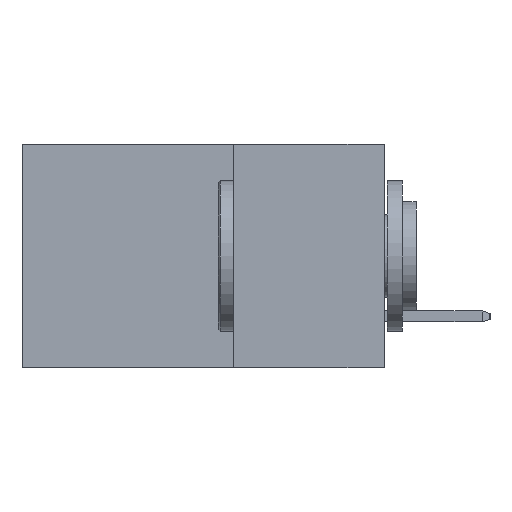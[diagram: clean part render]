
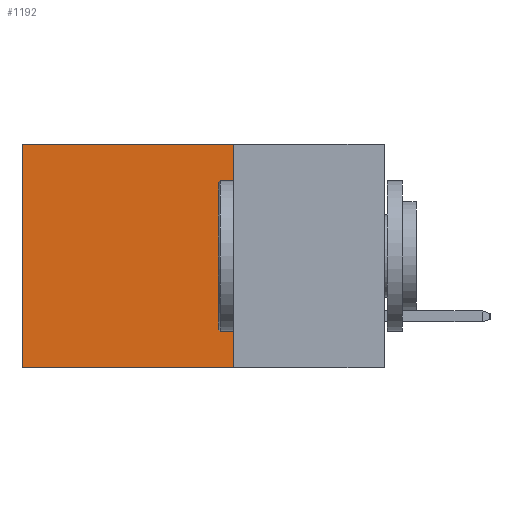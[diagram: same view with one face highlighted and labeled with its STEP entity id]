
A CAD part, left-side view. The second image highlights one B-rep face of the part: STEP entity #1192.
In plain terms, the highlighted planar face has unit normal (-1, 0, 0).
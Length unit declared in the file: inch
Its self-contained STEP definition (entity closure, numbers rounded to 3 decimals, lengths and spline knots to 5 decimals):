
#42 = CARTESIAN_POINT ( 'NONE',  ( 0.2615, 0.25, 0. ) ) ;
#77 = DIRECTION ( 'NONE',  ( 0., 1., 0. ) ) ;
#225 = ORIENTED_EDGE ( 'NONE', *, *, #9653, .T. ) ;
#445 = ORIENTED_EDGE ( 'NONE', *, *, #18104, .T. ) ;
#1060 = VECTOR ( 'NONE', #6562, 39.37008 ) ;
#1101 = CARTESIAN_POINT ( 'NONE',  ( 0.2615, 0.6, 0. ) ) ;
#1192 = ADVANCED_FACE ( 'NONE', ( #12838 ), #11762, .F. ) ;
#1375 = CARTESIAN_POINT ( 'NONE',  ( 0.2615, 0.25, -0.37 ) ) ;
#1571 = ORIENTED_EDGE ( 'NONE', *, *, #18103, .F. ) ;
#1589 = VERTEX_POINT ( 'NONE', #2578 ) ;
#2191 = AXIS2_PLACEMENT_3D ( 'NONE', #11830, #11569, #11437 ) ;
#2578 = CARTESIAN_POINT ( 'NONE',  ( 0.2615, 0.25, 0. ) ) ;
#3271 = VECTOR ( 'NONE', #77, 39.37008 ) ;
#4310 = VERTEX_POINT ( 'NONE', #17170 ) ;
#4806 = CARTESIAN_POINT ( 'NONE',  ( 0.2615, 0.6, -0.37 ) ) ;
#6152 = LINE ( 'NONE', #1375, #10153 ) ;
#6253 = DIRECTION ( 'NONE',  ( 0., 1., 0. ) ) ;
#6562 = DIRECTION ( 'NONE',  ( 0., 0., -1. ) ) ;
#6705 = CARTESIAN_POINT ( 'NONE',  ( 0.2615, 0.25, -0.37 ) ) ;
#7141 = VERTEX_POINT ( 'NONE', #1101 ) ;
#9653 = EDGE_CURVE ( 'NONE', #1589, #7141, #12821, .T. ) ;
#10153 = VECTOR ( 'NONE', #13186, 39.37008 ) ;
#11437 = DIRECTION ( 'NONE',  ( 0., 0., -1. ) ) ;
#11569 = DIRECTION ( 'NONE',  ( 1., 0., 0. ) ) ;
#11762 = PLANE ( 'NONE',  #2191 ) ;
#11830 = CARTESIAN_POINT ( 'NONE',  ( 0.2615, 0.25, -0.37 ) ) ;
#12821 = LINE ( 'NONE', #42, #3271 ) ;
#12838 = FACE_OUTER_BOUND ( 'NONE', #16505, .T. ) ;
#13186 = DIRECTION ( 'NONE',  ( 0., 0., -1. ) ) ;
#13377 = CARTESIAN_POINT ( 'NONE',  ( 0.2615, 0.6, -0.37 ) ) ;
#14423 = EDGE_CURVE ( 'NONE', #4310, #18855, #20795, .T. ) ;
#16505 = EDGE_LOOP ( 'NONE', ( #445, #16764, #1571, #225 ) ) ;
#16764 = ORIENTED_EDGE ( 'NONE', *, *, #14423, .F. ) ;
#17170 = CARTESIAN_POINT ( 'NONE',  ( 0.2615, 0.25, -0.37 ) ) ;
#18103 = EDGE_CURVE ( 'NONE', #1589, #4310, #6152, .T. ) ;
#18104 = EDGE_CURVE ( 'NONE', #7141, #18855, #19369, .T. ) ;
#18771 = VECTOR ( 'NONE', #6253, 39.37008 ) ;
#18855 = VERTEX_POINT ( 'NONE', #13377 ) ;
#19369 = LINE ( 'NONE', #4806, #1060 ) ;
#20795 = LINE ( 'NONE', #6705, #18771 ) ;
